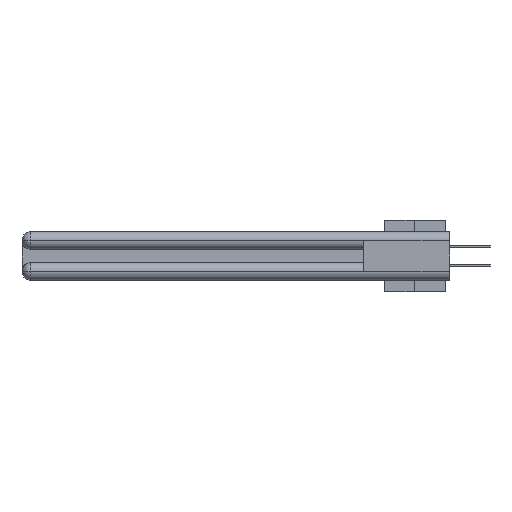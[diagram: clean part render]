
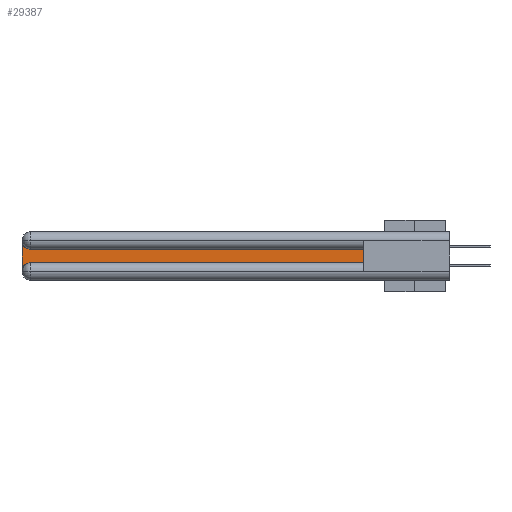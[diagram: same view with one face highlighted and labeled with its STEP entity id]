
A CAD part, left-side view. The second image highlights one B-rep face of the part: STEP entity #29387.
In plain terms, the highlighted planar face has unit normal (-1, 0, 0).
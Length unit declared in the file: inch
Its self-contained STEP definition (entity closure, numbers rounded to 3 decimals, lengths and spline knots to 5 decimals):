
#1107 = CARTESIAN_POINT ( 'NONE',  ( 0.075, 0.6, -0.1225 ) ) ;
#1147 = FACE_OUTER_BOUND ( 'NONE', #29003, .T. ) ;
#3702 = CARTESIAN_POINT ( 'NONE',  ( 0.075, 0.6, -0.2175 ) ) ;
#4421 = VERTEX_POINT ( 'NONE', #32387 ) ;
#4637 = VECTOR ( 'NONE', #20953, 39.37008 ) ;
#4656 = DIRECTION ( 'NONE',  ( 0., 1., 0. ) ) ;
#5834 = ORIENTED_EDGE ( 'NONE', *, *, #21086, .T. ) ;
#7961 = AXIS2_PLACEMENT_3D ( 'NONE', #20226, #9952, #16999 ) ;
#8104 = ORIENTED_EDGE ( 'NONE', *, *, #28966, .T. ) ;
#8251 = VECTOR ( 'NONE', #4656, 39.37008 ) ;
#9952 = DIRECTION ( 'NONE',  ( 1., 0., 0. ) ) ;
#10443 = DIRECTION ( 'NONE',  ( 1., 0., 0. ) ) ;
#11577 = LINE ( 'NONE', #28014, #24202 ) ;
#12843 = ORIENTED_EDGE ( 'NONE', *, *, #22012, .T. ) ;
#12976 = PLANE ( 'NONE',  #15006 ) ;
#13394 = DIRECTION ( 'NONE',  ( 0., 0., -1. ) ) ;
#13977 = CARTESIAN_POINT ( 'NONE',  ( 0.075, 2.94, -0.2775 ) ) ;
#15006 = AXIS2_PLACEMENT_3D ( 'NONE', #37063, #18813, #41043 ) ;
#15039 = LINE ( 'NONE', #27651, #4637 ) ;
#15318 = CIRCLE ( 'NONE', #7961, 0.06 ) ;
#16999 = DIRECTION ( 'NONE',  ( 0., 0., -1. ) ) ;
#18813 = DIRECTION ( 'NONE',  ( 1., 0., 0. ) ) ;
#18938 = VERTEX_POINT ( 'NONE', #20437 ) ;
#20226 = CARTESIAN_POINT ( 'NONE',  ( 0.075, 2.94, -0.0625 ) ) ;
#20437 = CARTESIAN_POINT ( 'NONE',  ( 0.075, 2.94, -0.1225 ) ) ;
#20953 = DIRECTION ( 'NONE',  ( 0., 0., 1. ) ) ;
#21086 = EDGE_CURVE ( 'NONE', #38013, #42577, #30944, .T. ) ;
#22012 = EDGE_CURVE ( 'NONE', #31809, #33610, #15039, .T. ) ;
#22651 = CARTESIAN_POINT ( 'NONE',  ( 0.075, 3., -0.2775 ) ) ;
#24202 = VECTOR ( 'NONE', #13394, 39.37008 ) ;
#24379 = DIRECTION ( 'NONE',  ( 0., 0., -1. ) ) ;
#24789 = DIRECTION ( 'NONE',  ( 0., -1., 0. ) ) ;
#27620 = ORIENTED_EDGE ( 'NONE', *, *, #29056, .T. ) ;
#27651 = CARTESIAN_POINT ( 'NONE',  ( 0.075, 0.6, -0.2175 ) ) ;
#27810 = EDGE_CURVE ( 'NONE', #4421, #38013, #11577, .T. ) ;
#28014 = CARTESIAN_POINT ( 'NONE',  ( 0.075, 3., -0.2175 ) ) ;
#28472 = CARTESIAN_POINT ( 'NONE',  ( 0.075, 0.6, -0.1225 ) ) ;
#28966 = EDGE_CURVE ( 'NONE', #18938, #4421, #15318, .T. ) ;
#28986 = LINE ( 'NONE', #1107, #8251 ) ;
#29003 = EDGE_LOOP ( 'NONE', ( #37394, #8104, #32010, #5834, #27620, #12843 ) ) ;
#29056 = EDGE_CURVE ( 'NONE', #42577, #31809, #35438, .T. ) ;
#29387 = ADVANCED_FACE ( 'NONE', ( #1147 ), #12976, .F. ) ;
#30502 = EDGE_CURVE ( 'NONE', #33610, #18938, #28986, .T. ) ;
#30944 = CIRCLE ( 'NONE', #39541, 0.06 ) ;
#31640 = CARTESIAN_POINT ( 'NONE',  ( 0.075, 2.94, -0.2175 ) ) ;
#31809 = VERTEX_POINT ( 'NONE', #35461 ) ;
#32010 = ORIENTED_EDGE ( 'NONE', *, *, #27810, .T. ) ;
#32387 = CARTESIAN_POINT ( 'NONE',  ( 0.075, 3., -0.0625 ) ) ;
#33274 = VECTOR ( 'NONE', #24789, 39.37008 ) ;
#33610 = VERTEX_POINT ( 'NONE', #28472 ) ;
#35438 = LINE ( 'NONE', #3702, #33274 ) ;
#35461 = CARTESIAN_POINT ( 'NONE',  ( 0.075, 0.6, -0.2175 ) ) ;
#37063 = CARTESIAN_POINT ( 'NONE',  ( 0.075, 3., -0.1225 ) ) ;
#37394 = ORIENTED_EDGE ( 'NONE', *, *, #30502, .T. ) ;
#38013 = VERTEX_POINT ( 'NONE', #22651 ) ;
#39541 = AXIS2_PLACEMENT_3D ( 'NONE', #13977, #10443, #24379 ) ;
#41043 = DIRECTION ( 'NONE',  ( 0., 0., -1. ) ) ;
#42577 = VERTEX_POINT ( 'NONE', #31640 ) ;
